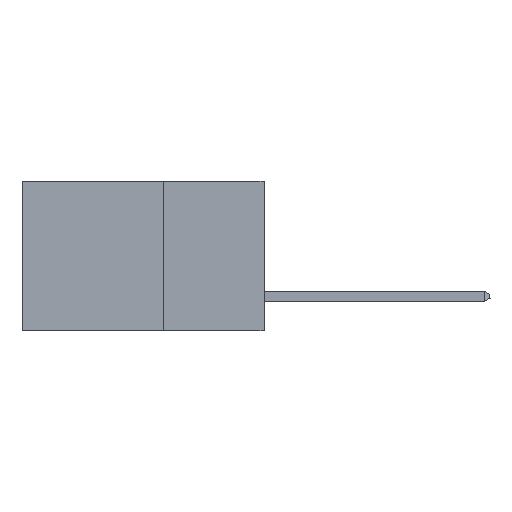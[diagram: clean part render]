
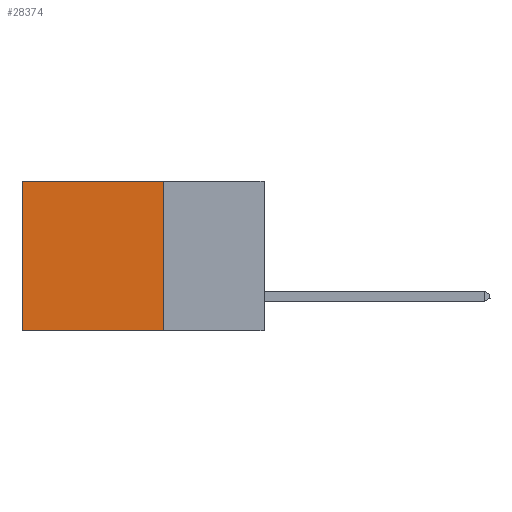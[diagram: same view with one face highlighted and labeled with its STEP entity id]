
A CAD part, left-side view. The second image highlights one B-rep face of the part: STEP entity #28374.
In plain terms, the highlighted planar face has unit normal (-1, 0, 0).
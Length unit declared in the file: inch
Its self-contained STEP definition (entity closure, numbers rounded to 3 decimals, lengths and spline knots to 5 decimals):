
#575 = VECTOR ( 'NONE', #5521, 39.37008 ) ;
#947 = DIRECTION ( 'NONE',  ( 0., 0., -1. ) ) ;
#1577 = PLANE ( 'NONE',  #19229 ) ;
#1723 = DIRECTION ( 'NONE',  ( 0., 1., 0. ) ) ;
#2891 = CARTESIAN_POINT ( 'NONE',  ( 0.298, 0.25, -0.37 ) ) ;
#3318 = ORIENTED_EDGE ( 'NONE', *, *, #14450, .T. ) ;
#5521 = DIRECTION ( 'NONE',  ( 0., 0., -1. ) ) ;
#6035 = LINE ( 'NONE', #8140, #25253 ) ;
#6953 = ORIENTED_EDGE ( 'NONE', *, *, #14455, .F. ) ;
#7507 = VERTEX_POINT ( 'NONE', #2891 ) ;
#7785 = ORIENTED_EDGE ( 'NONE', *, *, #11498, .F. ) ;
#7897 = VECTOR ( 'NONE', #29188, 39.37008 ) ;
#8140 = CARTESIAN_POINT ( 'NONE',  ( 0.298, 0.6, 0. ) ) ;
#8643 = CARTESIAN_POINT ( 'NONE',  ( 0.298, 0.25, -0.37 ) ) ;
#8772 = DIRECTION ( 'NONE',  ( 1., 0., 0. ) ) ;
#9586 = CARTESIAN_POINT ( 'NONE',  ( 0.298, 0.25, 0. ) ) ;
#9759 = LINE ( 'NONE', #8643, #7897 ) ;
#10311 = CARTESIAN_POINT ( 'NONE',  ( 0.298, 0.25, 0. ) ) ;
#10748 = VERTEX_POINT ( 'NONE', #18284 ) ;
#11498 = EDGE_CURVE ( 'NONE', #7507, #10748, #9759, .T. ) ;
#11832 = VERTEX_POINT ( 'NONE', #13033 ) ;
#13033 = CARTESIAN_POINT ( 'NONE',  ( 0.298, 0.6, 0. ) ) ;
#13499 = DIRECTION ( 'NONE',  ( 0., 0., -1. ) ) ;
#14450 = EDGE_CURVE ( 'NONE', #11832, #10748, #6035, .T. ) ;
#14455 = EDGE_CURVE ( 'NONE', #18769, #7507, #25947, .T. ) ;
#14468 = EDGE_LOOP ( 'NONE', ( #3318, #7785, #6953, #25221 ) ) ;
#15723 = CARTESIAN_POINT ( 'NONE',  ( 0.298, 0.25, 0. ) ) ;
#18284 = CARTESIAN_POINT ( 'NONE',  ( 0.298, 0.6, -0.37 ) ) ;
#18769 = VERTEX_POINT ( 'NONE', #9586 ) ;
#19229 = AXIS2_PLACEMENT_3D ( 'NONE', #15723, #8772, #13499 ) ;
#22123 = FACE_OUTER_BOUND ( 'NONE', #14468, .T. ) ;
#22594 = VECTOR ( 'NONE', #1723, 39.37008 ) ;
#24757 = CARTESIAN_POINT ( 'NONE',  ( 0.298, 0.25, 0. ) ) ;
#25221 = ORIENTED_EDGE ( 'NONE', *, *, #26933, .T. ) ;
#25253 = VECTOR ( 'NONE', #947, 39.37008 ) ;
#25486 = LINE ( 'NONE', #24757, #22594 ) ;
#25947 = LINE ( 'NONE', #10311, #575 ) ;
#26933 = EDGE_CURVE ( 'NONE', #18769, #11832, #25486, .T. ) ;
#28374 = ADVANCED_FACE ( 'NONE', ( #22123 ), #1577, .F. ) ;
#29188 = DIRECTION ( 'NONE',  ( 0., 1., 0. ) ) ;
